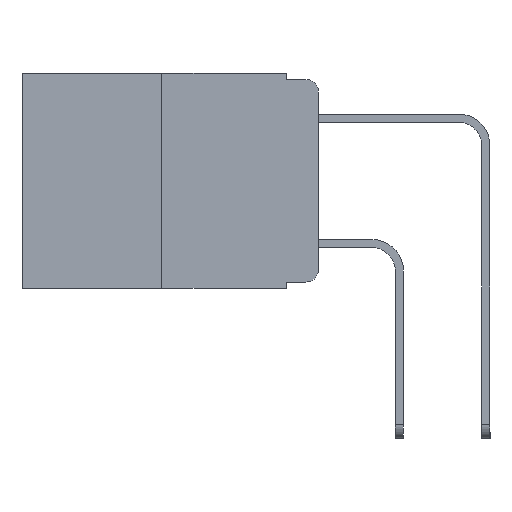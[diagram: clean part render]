
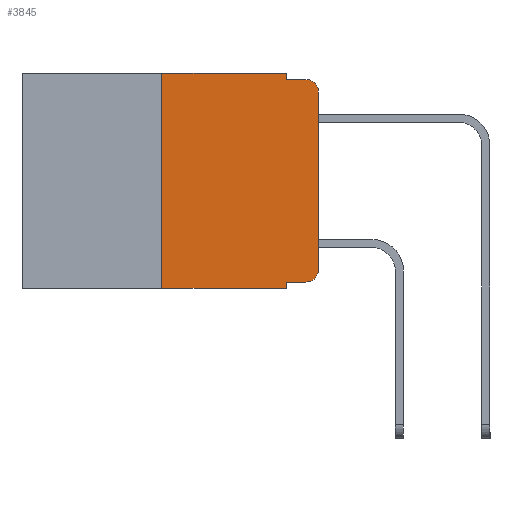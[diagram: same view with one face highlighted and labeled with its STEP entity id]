
A CAD part, left-side view. The second image highlights one B-rep face of the part: STEP entity #3845.
In plain terms, the highlighted planar face has unit normal (-1, 0, 0).
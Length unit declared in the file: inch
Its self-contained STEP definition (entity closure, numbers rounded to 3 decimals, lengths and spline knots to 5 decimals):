
#475 = ORIENTED_EDGE ( 'NONE', *, *, #22268, .F. ) ;
#578 = CARTESIAN_POINT ( 'NONE',  ( 0., 0.473, 0. ) ) ;
#1302 = ORIENTED_EDGE ( 'NONE', *, *, #7954, .F. ) ;
#1466 = VECTOR ( 'NONE', #18191, 39.37008 ) ;
#2042 = LINE ( 'NONE', #21605, #1466 ) ;
#2544 = DIRECTION ( 'NONE',  ( 0., 0., 1. ) ) ;
#3215 = CARTESIAN_POINT ( 'NONE',  ( 0., 0.051, 0. ) ) ;
#3393 = EDGE_CURVE ( 'NONE', #19387, #11124, #18951, .T. ) ;
#3487 = CARTESIAN_POINT ( 'NONE',  ( 0., 0.02, -0.03 ) ) ;
#3845 = ADVANCED_FACE ( 'NONE', ( #18927 ), #4698, .F. ) ;
#4291 = VERTEX_POINT ( 'NONE', #9865 ) ;
#4621 = CARTESIAN_POINT ( 'NONE',  ( 0., 0.473, -0.343 ) ) ;
#4640 = CARTESIAN_POINT ( 'NONE',  ( 0., 0.02, -0.333 ) ) ;
#4698 = PLANE ( 'NONE',  #10131 ) ;
#4768 = AXIS2_PLACEMENT_3D ( 'NONE', #6775, #19304, #8533 ) ;
#5267 = DIRECTION ( 'NONE',  ( 0., 0., -1. ) ) ;
#5529 = LINE ( 'NONE', #12949, #22774 ) ;
#5554 = CARTESIAN_POINT ( 'NONE',  ( 0., 0.051, 0. ) ) ;
#6046 = EDGE_CURVE ( 'NONE', #19658, #14489, #5529, .T. ) ;
#6135 = DIRECTION ( 'NONE',  ( 0., -1., 0. ) ) ;
#6499 = DIRECTION ( 'NONE',  ( 0., 0., -1. ) ) ;
#6526 = DIRECTION ( 'NONE',  ( 0., -1., 0. ) ) ;
#6775 = CARTESIAN_POINT ( 'NONE',  ( 0., 0.02, -0.313 ) ) ;
#6817 = LINE ( 'NONE', #3215, #16405 ) ;
#7191 = EDGE_CURVE ( 'NONE', #14207, #14962, #18374, .T. ) ;
#7520 = EDGE_CURVE ( 'NONE', #8707, #11124, #2042, .T. ) ;
#7954 = EDGE_CURVE ( 'NONE', #4291, #8707, #6817, .T. ) ;
#8055 = VERTEX_POINT ( 'NONE', #19466 ) ;
#8533 = DIRECTION ( 'NONE',  ( 0., 0., -1. ) ) ;
#8707 = VERTEX_POINT ( 'NONE', #21263 ) ;
#8910 = CARTESIAN_POINT ( 'NONE',  ( 0., 0.25, -0.343 ) ) ;
#9646 = EDGE_CURVE ( 'NONE', #19658, #20314, #20700, .T. ) ;
#9865 = CARTESIAN_POINT ( 'NONE',  ( 0., 0.051, 0. ) ) ;
#10131 = AXIS2_PLACEMENT_3D ( 'NONE', #22435, #17254, #6499 ) ;
#11124 = VERTEX_POINT ( 'NONE', #22755 ) ;
#11451 = EDGE_CURVE ( 'NONE', #8055, #19387, #13711, .T. ) ;
#11500 = CARTESIAN_POINT ( 'NONE',  ( 0., 0., 0. ) ) ;
#11783 = VECTOR ( 'NONE', #15385, 39.37008 ) ;
#12144 = CARTESIAN_POINT ( 'NONE',  ( 0., 0.25, 0. ) ) ;
#12174 = DIRECTION ( 'NONE',  ( 0., 0., -1. ) ) ;
#12579 = VECTOR ( 'NONE', #2544, 39.37008 ) ;
#12787 = EDGE_CURVE ( 'NONE', #14489, #4291, #22004, .T. ) ;
#12949 = CARTESIAN_POINT ( 'NONE',  ( 0., 0.25, 0. ) ) ;
#13585 = VECTOR ( 'NONE', #6526, 39.37008 ) ;
#13697 = ORIENTED_EDGE ( 'NONE', *, *, #9646, .T. ) ;
#13700 = CIRCLE ( 'NONE', #4768, 0.02 ) ;
#13711 = LINE ( 'NONE', #11500, #12579 ) ;
#14207 = VERTEX_POINT ( 'NONE', #18773 ) ;
#14489 = VERTEX_POINT ( 'NONE', #12144 ) ;
#14545 = ORIENTED_EDGE ( 'NONE', *, *, #7520, .F. ) ;
#14962 = VERTEX_POINT ( 'NONE', #4640 ) ;
#15385 = DIRECTION ( 'NONE',  ( 0., -1., 0. ) ) ;
#16005 = ORIENTED_EDGE ( 'NONE', *, *, #20787, .T. ) ;
#16050 = DIRECTION ( 'NONE',  ( -1., 0., 0. ) ) ;
#16331 = CARTESIAN_POINT ( 'NONE',  ( 0., 0.051, -0.343 ) ) ;
#16405 = VECTOR ( 'NONE', #12174, 39.37008 ) ;
#17254 = DIRECTION ( 'NONE',  ( 1., 0., 0. ) ) ;
#17283 = CARTESIAN_POINT ( 'NONE',  ( 0., 0.051, -0.333 ) ) ;
#17375 = VECTOR ( 'NONE', #6135, 39.37008 ) ;
#17636 = ORIENTED_EDGE ( 'NONE', *, *, #11451, .T. ) ;
#18191 = DIRECTION ( 'NONE',  ( 0., -1., 0. ) ) ;
#18282 = AXIS2_PLACEMENT_3D ( 'NONE', #3487, #16050, #5267 ) ;
#18311 = DIRECTION ( 'NONE',  ( 0., 0., 1. ) ) ;
#18374 = LINE ( 'NONE', #17283, #13585 ) ;
#18682 = LINE ( 'NONE', #5554, #22750 ) ;
#18773 = CARTESIAN_POINT ( 'NONE',  ( 0., 0.051, -0.333 ) ) ;
#18927 = FACE_OUTER_BOUND ( 'NONE', #20870, .T. ) ;
#18951 = CIRCLE ( 'NONE', #18282, 0.02 ) ;
#19304 = DIRECTION ( 'NONE',  ( -1., 0., 0. ) ) ;
#19387 = VERTEX_POINT ( 'NONE', #22320 ) ;
#19466 = CARTESIAN_POINT ( 'NONE',  ( 0., 0., -0.313 ) ) ;
#19568 = ORIENTED_EDGE ( 'NONE', *, *, #7191, .T. ) ;
#19658 = VERTEX_POINT ( 'NONE', #8910 ) ;
#19852 = DIRECTION ( 'NONE',  ( 0., 0., -1. ) ) ;
#20314 = VERTEX_POINT ( 'NONE', #16331 ) ;
#20700 = LINE ( 'NONE', #4621, #11783 ) ;
#20787 = EDGE_CURVE ( 'NONE', #14962, #8055, #13700, .T. ) ;
#20870 = EDGE_LOOP ( 'NONE', ( #17636, #22812, #14545, #1302, #20911, #22006, #13697, #475, #19568, #16005 ) ) ;
#20911 = ORIENTED_EDGE ( 'NONE', *, *, #12787, .F. ) ;
#21263 = CARTESIAN_POINT ( 'NONE',  ( 0., 0.051, -0.01 ) ) ;
#21605 = CARTESIAN_POINT ( 'NONE',  ( 0., 0.051, -0.01 ) ) ;
#22004 = LINE ( 'NONE', #578, #17375 ) ;
#22006 = ORIENTED_EDGE ( 'NONE', *, *, #6046, .F. ) ;
#22268 = EDGE_CURVE ( 'NONE', #14207, #20314, #18682, .T. ) ;
#22320 = CARTESIAN_POINT ( 'NONE',  ( 0., 0., -0.03 ) ) ;
#22435 = CARTESIAN_POINT ( 'NONE',  ( 0., 0.473, 0. ) ) ;
#22750 = VECTOR ( 'NONE', #19852, 39.37008 ) ;
#22755 = CARTESIAN_POINT ( 'NONE',  ( 0., 0.02, -0.01 ) ) ;
#22774 = VECTOR ( 'NONE', #18311, 39.37008 ) ;
#22812 = ORIENTED_EDGE ( 'NONE', *, *, #3393, .T. ) ;
